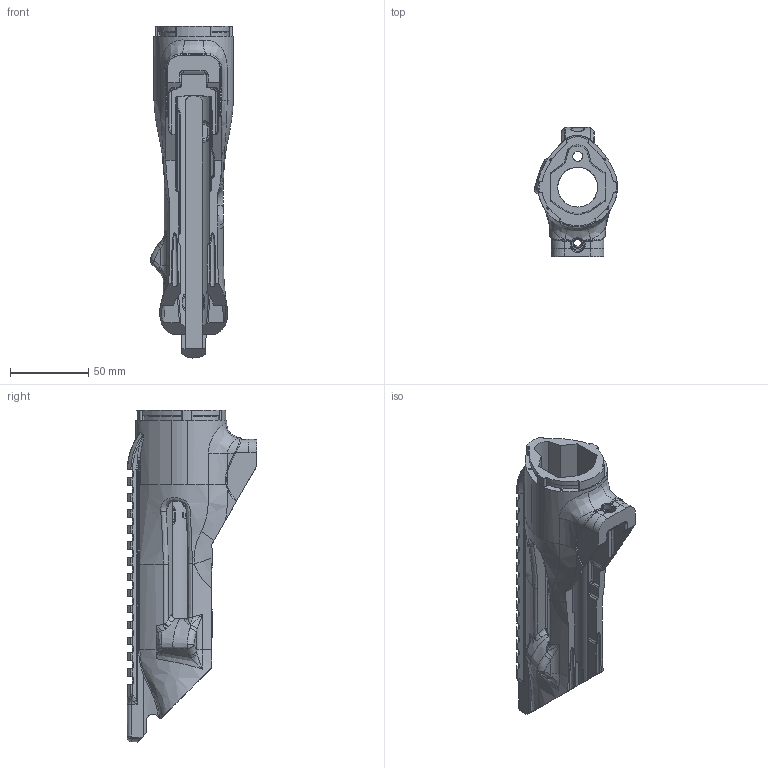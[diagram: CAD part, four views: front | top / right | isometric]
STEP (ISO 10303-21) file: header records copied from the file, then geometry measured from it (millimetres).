
FILE_DESCRIPTION (( 'STEP AP203' ), '1' );
FILE_NAME ('Orca Upper V5.3.STEP', '2023-01-20T23:40:11', ( '' ), ( '' ), 'SwSTEP 2.0', 'SolidWorks 2021', '' );
FILE_SCHEMA (( 'CONFIG_CONTROL_DESIGN' ));
Length unit declared in the file: inch
Products named in the file (1): Orca Upper V5.3
Bounding box: 53 x 82.47 x 212.07 mm (x, y, z)
Volume: 192055.7 mm3; surface area: 59796 mm2
Topology: 1 solids, 1 shells, 937 faces, 2496 edges, 1531 vertices
Faces by surface type: bspline 387, cylinder 277, plane 235, torus 17, sphere 16, cone 5
Entity records: 64258 total; most frequent: CARTESIAN_POINT 44389, ORIENTED_EDGE 4924, DIRECTION 3138, EDGE_CURVE 2462, VERTEX_POINT 1531, AXIS2_PLACEMENT_3D 1176, EDGE_LOOP 949, FACE_OUTER_BOUND 937
